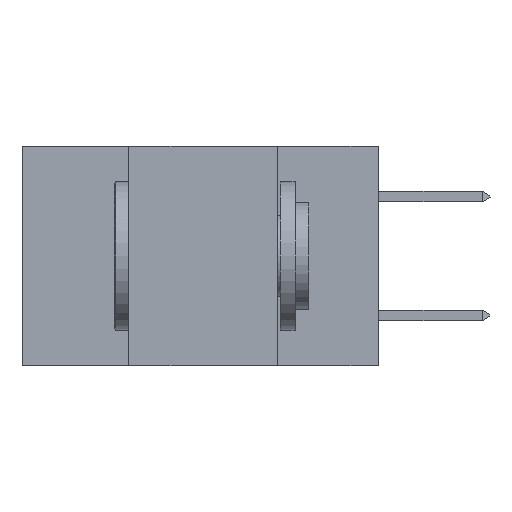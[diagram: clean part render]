
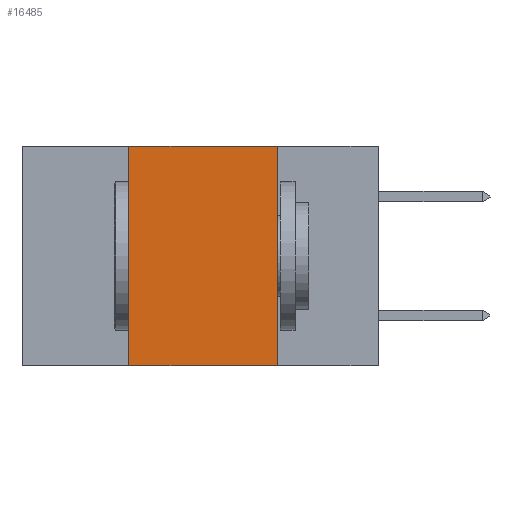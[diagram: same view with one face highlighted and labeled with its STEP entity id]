
A CAD part, left-side view. The second image highlights one B-rep face of the part: STEP entity #16485.
In plain terms, the highlighted planar face has unit normal (-1, 0, 0).
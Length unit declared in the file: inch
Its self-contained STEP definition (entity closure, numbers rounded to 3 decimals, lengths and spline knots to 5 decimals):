
#168 = LINE ( 'NONE', #11919, #16950 ) ;
#718 = LINE ( 'NONE', #20074, #14454 ) ;
#1089 = VERTEX_POINT ( 'NONE', #2824 ) ;
#2221 = EDGE_CURVE ( 'NONE', #20186, #1089, #168, .T. ) ;
#2824 = CARTESIAN_POINT ( 'NONE',  ( 0., 0.17, -0.37 ) ) ;
#3860 = FACE_OUTER_BOUND ( 'NONE', #12877, .T. ) ;
#4393 = CARTESIAN_POINT ( 'NONE',  ( 0., 0.6, 0. ) ) ;
#5783 = AXIS2_PLACEMENT_3D ( 'NONE', #15646, #19140, #10321 ) ;
#6889 = PLANE ( 'NONE',  #5783 ) ;
#7525 = DIRECTION ( 'NONE',  ( 0., 0., 1. ) ) ;
#7584 = LINE ( 'NONE', #17707, #17075 ) ;
#7854 = VECTOR ( 'NONE', #11647, 39.37008 ) ;
#10004 = ORIENTED_EDGE ( 'NONE', *, *, #2221, .F. ) ;
#10321 = DIRECTION ( 'NONE',  ( 0., 0., -1. ) ) ;
#11158 = ORIENTED_EDGE ( 'NONE', *, *, #22150, .T. ) ;
#11597 = ORIENTED_EDGE ( 'NONE', *, *, #15249, .F. ) ;
#11647 = DIRECTION ( 'NONE',  ( 0., -1., 0. ) ) ;
#11783 = ORIENTED_EDGE ( 'NONE', *, *, #12285, .F. ) ;
#11919 = CARTESIAN_POINT ( 'NONE',  ( 0., 0.17, 0. ) ) ;
#12285 = EDGE_CURVE ( 'NONE', #15324, #20186, #12883, .T. ) ;
#12877 = EDGE_LOOP ( 'NONE', ( #10004, #11783, #11597, #11158 ) ) ;
#12883 = LINE ( 'NONE', #4393, #7854 ) ;
#14168 = CARTESIAN_POINT ( 'NONE',  ( 0., 0.42, -0.37 ) ) ;
#14454 = VECTOR ( 'NONE', #7525, 39.37008 ) ;
#15249 = EDGE_CURVE ( 'NONE', #16616, #15324, #718, .T. ) ;
#15324 = VERTEX_POINT ( 'NONE', #16507 ) ;
#15646 = CARTESIAN_POINT ( 'NONE',  ( 0., 0.6, 0. ) ) ;
#16485 = ADVANCED_FACE ( 'NONE', ( #3860 ), #6889, .F. ) ;
#16507 = CARTESIAN_POINT ( 'NONE',  ( 0., 0.42, 0. ) ) ;
#16616 = VERTEX_POINT ( 'NONE', #14168 ) ;
#16950 = VECTOR ( 'NONE', #21052, 39.37008 ) ;
#17075 = VECTOR ( 'NONE', #17559, 39.37008 ) ;
#17559 = DIRECTION ( 'NONE',  ( 0., -1., 0. ) ) ;
#17707 = CARTESIAN_POINT ( 'NONE',  ( 0., 0.6, -0.37 ) ) ;
#17794 = CARTESIAN_POINT ( 'NONE',  ( 0., 0.17, 0. ) ) ;
#19140 = DIRECTION ( 'NONE',  ( 1., 0., 0. ) ) ;
#20074 = CARTESIAN_POINT ( 'NONE',  ( 0., 0.42, 0. ) ) ;
#20186 = VERTEX_POINT ( 'NONE', #17794 ) ;
#21052 = DIRECTION ( 'NONE',  ( 0., 0., -1. ) ) ;
#22150 = EDGE_CURVE ( 'NONE', #16616, #1089, #7584, .T. ) ;
